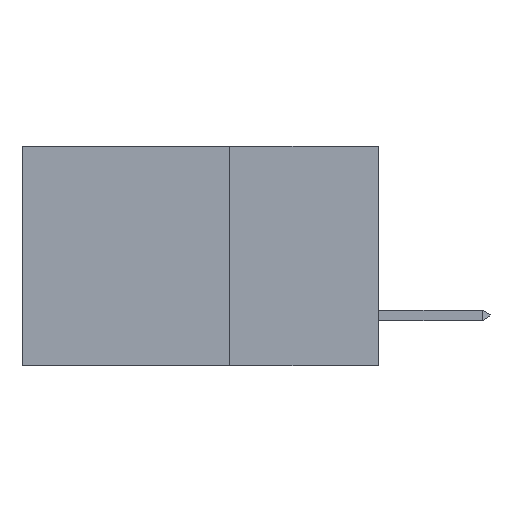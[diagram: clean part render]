
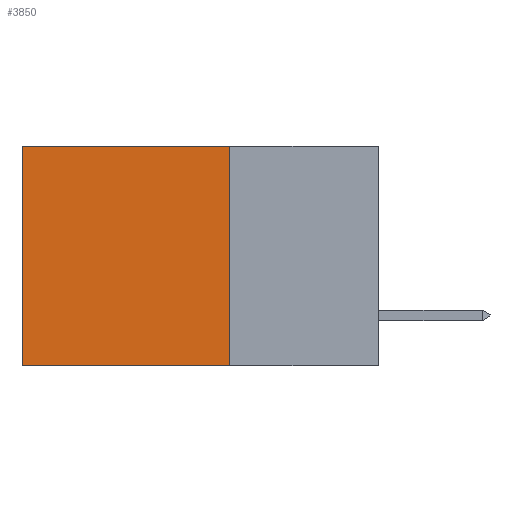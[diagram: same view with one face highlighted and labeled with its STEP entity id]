
A CAD part, left-side view. The second image highlights one B-rep face of the part: STEP entity #3850.
In plain terms, the highlighted planar face has unit normal (-1, 0, 0).
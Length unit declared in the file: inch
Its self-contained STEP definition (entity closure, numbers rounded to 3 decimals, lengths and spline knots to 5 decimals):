
#16 = LINE ( 'NONE', #10896, #6538 ) ;
#491 = CARTESIAN_POINT ( 'NONE',  ( 0.2615, 0.6, -0.37 ) ) ;
#1094 = ORIENTED_EDGE ( 'NONE', *, *, #6602, .T. ) ;
#1275 = VERTEX_POINT ( 'NONE', #5369 ) ;
#2772 = EDGE_CURVE ( 'NONE', #9834, #8345, #10929, .T. ) ;
#3243 = VERTEX_POINT ( 'NONE', #491 ) ;
#3845 = PLANE ( 'NONE',  #8435 ) ;
#3850 = ADVANCED_FACE ( 'NONE', ( #7971 ), #3845, .F. ) ;
#5109 = CARTESIAN_POINT ( 'NONE',  ( 0.2615, 0.25, 0. ) ) ;
#5369 = CARTESIAN_POINT ( 'NONE',  ( 0.2615, 0.6, 0. ) ) ;
#5570 = EDGE_CURVE ( 'NONE', #1275, #3243, #6752, .T. ) ;
#6047 = DIRECTION ( 'NONE',  ( 1., 0., 0. ) ) ;
#6054 = ORIENTED_EDGE ( 'NONE', *, *, #2772, .F. ) ;
#6538 = VECTOR ( 'NONE', #7560, 39.37008 ) ;
#6602 = EDGE_CURVE ( 'NONE', #9834, #1275, #7509, .T. ) ;
#6628 = DIRECTION ( 'NONE',  ( 0., 0., -1. ) ) ;
#6752 = LINE ( 'NONE', #13183, #13811 ) ;
#7509 = LINE ( 'NONE', #5109, #13056 ) ;
#7560 = DIRECTION ( 'NONE',  ( 0., 1., 0. ) ) ;
#7843 = DIRECTION ( 'NONE',  ( 0., 0., -1. ) ) ;
#7971 = FACE_OUTER_BOUND ( 'NONE', #10022, .T. ) ;
#8203 = ORIENTED_EDGE ( 'NONE', *, *, #5570, .T. ) ;
#8345 = VERTEX_POINT ( 'NONE', #11302 ) ;
#8435 = AXIS2_PLACEMENT_3D ( 'NONE', #12631, #6047, #11386 ) ;
#8916 = ORIENTED_EDGE ( 'NONE', *, *, #12766, .F. ) ;
#9834 = VERTEX_POINT ( 'NONE', #12027 ) ;
#10022 = EDGE_LOOP ( 'NONE', ( #8203, #8916, #6054, #1094 ) ) ;
#10073 = CARTESIAN_POINT ( 'NONE',  ( 0.2615, 0.25, -0.37 ) ) ;
#10896 = CARTESIAN_POINT ( 'NONE',  ( 0.2615, 0.25, -0.37 ) ) ;
#10929 = LINE ( 'NONE', #10073, #11968 ) ;
#11302 = CARTESIAN_POINT ( 'NONE',  ( 0.2615, 0.25, -0.37 ) ) ;
#11386 = DIRECTION ( 'NONE',  ( 0., 0., -1. ) ) ;
#11909 = DIRECTION ( 'NONE',  ( 0., 1., 0. ) ) ;
#11968 = VECTOR ( 'NONE', #7843, 39.37008 ) ;
#12027 = CARTESIAN_POINT ( 'NONE',  ( 0.2615, 0.25, 0. ) ) ;
#12631 = CARTESIAN_POINT ( 'NONE',  ( 0.2615, 0.25, -0.37 ) ) ;
#12766 = EDGE_CURVE ( 'NONE', #8345, #3243, #16, .T. ) ;
#13056 = VECTOR ( 'NONE', #11909, 39.37008 ) ;
#13183 = CARTESIAN_POINT ( 'NONE',  ( 0.2615, 0.6, -0.37 ) ) ;
#13811 = VECTOR ( 'NONE', #6628, 39.37008 ) ;
